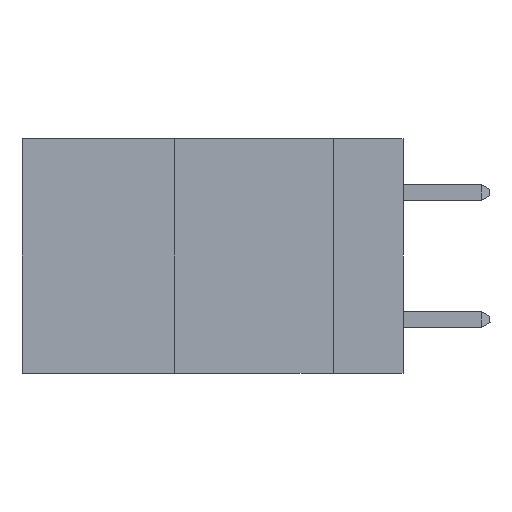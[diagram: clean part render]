
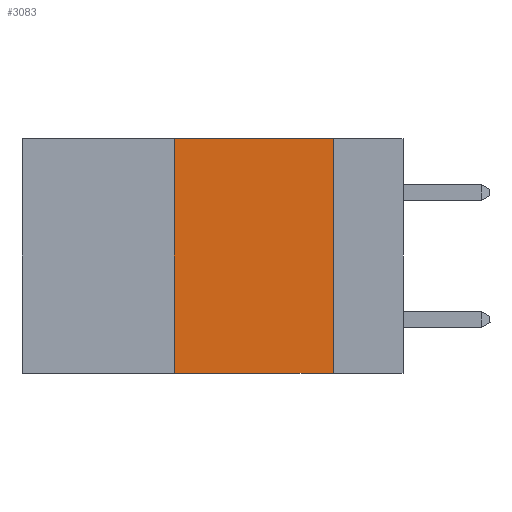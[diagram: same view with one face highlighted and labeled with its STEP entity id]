
A CAD part, left-side view. The second image highlights one B-rep face of the part: STEP entity #3083.
In plain terms, the highlighted planar face has unit normal (-1, 0, 0).
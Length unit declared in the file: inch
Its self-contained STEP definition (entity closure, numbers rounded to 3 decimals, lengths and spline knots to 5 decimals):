
#89 = ORIENTED_EDGE ( 'NONE', *, *, #9205, .F. ) ;
#94 = CARTESIAN_POINT ( 'NONE',  ( 0., 0.36, 0. ) ) ;
#163 = ORIENTED_EDGE ( 'NONE', *, *, #5907, .F. ) ;
#200 = ORIENTED_EDGE ( 'NONE', *, *, #6991, .F. ) ;
#404 = CARTESIAN_POINT ( 'NONE',  ( 0., 0.11, 0. ) ) ;
#552 = DIRECTION ( 'NONE',  ( 0., -1., 0. ) ) ;
#706 = ORIENTED_EDGE ( 'NONE', *, *, #8472, .T. ) ;
#722 = LINE ( 'NONE', #4633, #8903 ) ;
#958 = LINE ( 'NONE', #2763, #9111 ) ;
#1764 = CARTESIAN_POINT ( 'NONE',  ( 0., 0.36, -0.37 ) ) ;
#2152 = LINE ( 'NONE', #9855, #8204 ) ;
#2224 = CARTESIAN_POINT ( 'NONE',  ( 0., 0.6, 0. ) ) ;
#2237 = LINE ( 'NONE', #404, #6234 ) ;
#2414 = VERTEX_POINT ( 'NONE', #1764 ) ;
#2763 = CARTESIAN_POINT ( 'NONE',  ( 0., 0.6, -0.37 ) ) ;
#3066 = VERTEX_POINT ( 'NONE', #6921 ) ;
#3083 = ADVANCED_FACE ( 'NONE', ( #4510 ), #7743, .F. ) ;
#3850 = DIRECTION ( 'NONE',  ( 0., 0., -1. ) ) ;
#4310 = VERTEX_POINT ( 'NONE', #9112 ) ;
#4480 = DIRECTION ( 'NONE',  ( 0., 0., 1. ) ) ;
#4510 = FACE_OUTER_BOUND ( 'NONE', #8578, .T. ) ;
#4595 = AXIS2_PLACEMENT_3D ( 'NONE', #2224, #8528, #3850 ) ;
#4633 = CARTESIAN_POINT ( 'NONE',  ( 0., 0.6, 0. ) ) ;
#4732 = VERTEX_POINT ( 'NONE', #94 ) ;
#5907 = EDGE_CURVE ( 'NONE', #4732, #3066, #722, .T. ) ;
#6234 = VECTOR ( 'NONE', #7615, 39.37008 ) ;
#6921 = CARTESIAN_POINT ( 'NONE',  ( 0., 0.11, 0. ) ) ;
#6991 = EDGE_CURVE ( 'NONE', #2414, #4732, #2152, .T. ) ;
#7615 = DIRECTION ( 'NONE',  ( 0., 0., -1. ) ) ;
#7743 = PLANE ( 'NONE',  #4595 ) ;
#8204 = VECTOR ( 'NONE', #4480, 39.37008 ) ;
#8472 = EDGE_CURVE ( 'NONE', #2414, #4310, #958, .T. ) ;
#8528 = DIRECTION ( 'NONE',  ( 1., 0., 0. ) ) ;
#8578 = EDGE_LOOP ( 'NONE', ( #89, #163, #200, #706 ) ) ;
#8903 = VECTOR ( 'NONE', #552, 39.37008 ) ;
#9111 = VECTOR ( 'NONE', #9761, 39.37008 ) ;
#9112 = CARTESIAN_POINT ( 'NONE',  ( 0., 0.11, -0.37 ) ) ;
#9205 = EDGE_CURVE ( 'NONE', #3066, #4310, #2237, .T. ) ;
#9761 = DIRECTION ( 'NONE',  ( 0., -1., 0. ) ) ;
#9855 = CARTESIAN_POINT ( 'NONE',  ( 0., 0.36, 0. ) ) ;
